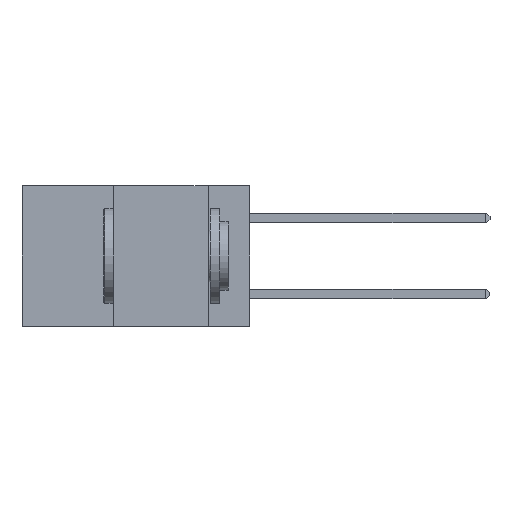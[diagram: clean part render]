
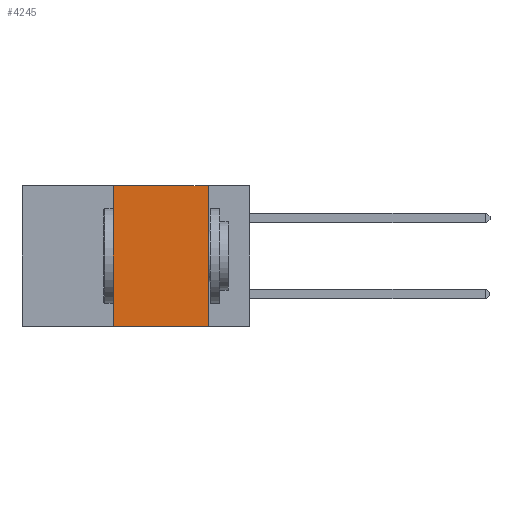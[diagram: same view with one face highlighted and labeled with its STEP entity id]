
A CAD part, left-side view. The second image highlights one B-rep face of the part: STEP entity #4245.
In plain terms, the highlighted planar face has unit normal (-1, 0, 0).
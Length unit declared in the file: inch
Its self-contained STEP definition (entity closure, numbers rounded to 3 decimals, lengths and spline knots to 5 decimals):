
#246 = CARTESIAN_POINT ( 'NONE',  ( 0., 0.11, -0.37 ) ) ;
#401 = DIRECTION ( 'NONE',  ( 0., 0., -1. ) ) ;
#532 = DIRECTION ( 'NONE',  ( 1., 0., 0. ) ) ;
#853 = CARTESIAN_POINT ( 'NONE',  ( 0., 0.6, -0.37 ) ) ;
#1138 = CARTESIAN_POINT ( 'NONE',  ( 0., 0.6, 0. ) ) ;
#1236 = PLANE ( 'NONE',  #7888 ) ;
#1429 = VECTOR ( 'NONE', #2829, 39.37008 ) ;
#1444 = VECTOR ( 'NONE', #10273, 39.37008 ) ;
#1738 = EDGE_LOOP ( 'NONE', ( #7374, #2840, #4292, #3475 ) ) ;
#2829 = DIRECTION ( 'NONE',  ( 0., 0., -1. ) ) ;
#2840 = ORIENTED_EDGE ( 'NONE', *, *, #3619, .F. ) ;
#3176 = VECTOR ( 'NONE', #3326, 39.37008 ) ;
#3211 = CARTESIAN_POINT ( 'NONE',  ( 0., 0.36, 0. ) ) ;
#3326 = DIRECTION ( 'NONE',  ( 0., -1., 0. ) ) ;
#3475 = ORIENTED_EDGE ( 'NONE', *, *, #9658, .T. ) ;
#3619 = EDGE_CURVE ( 'NONE', #6064, #11494, #4301, .T. ) ;
#3938 = VERTEX_POINT ( 'NONE', #13846 ) ;
#4157 = CARTESIAN_POINT ( 'NONE',  ( 0., 0.6, 0. ) ) ;
#4245 = ADVANCED_FACE ( 'NONE', ( #11407 ), #1236, .F. ) ;
#4252 = VERTEX_POINT ( 'NONE', #246 ) ;
#4292 = ORIENTED_EDGE ( 'NONE', *, *, #14094, .F. ) ;
#4301 = LINE ( 'NONE', #4157, #3176 ) ;
#4622 = LINE ( 'NONE', #853, #1444 ) ;
#6064 = VERTEX_POINT ( 'NONE', #11133 ) ;
#7374 = ORIENTED_EDGE ( 'NONE', *, *, #10111, .F. ) ;
#7888 = AXIS2_PLACEMENT_3D ( 'NONE', #1138, #532, #401 ) ;
#8120 = LINE ( 'NONE', #11054, #1429 ) ;
#9104 = DIRECTION ( 'NONE',  ( 0., 0., 1. ) ) ;
#9658 = EDGE_CURVE ( 'NONE', #3938, #4252, #4622, .T. ) ;
#10111 = EDGE_CURVE ( 'NONE', #11494, #4252, #8120, .T. ) ;
#10273 = DIRECTION ( 'NONE',  ( 0., -1., 0. ) ) ;
#10345 = LINE ( 'NONE', #3211, #12935 ) ;
#10732 = CARTESIAN_POINT ( 'NONE',  ( 0., 0.11, 0. ) ) ;
#11054 = CARTESIAN_POINT ( 'NONE',  ( 0., 0.11, 0. ) ) ;
#11133 = CARTESIAN_POINT ( 'NONE',  ( 0., 0.36, 0. ) ) ;
#11407 = FACE_OUTER_BOUND ( 'NONE', #1738, .T. ) ;
#11494 = VERTEX_POINT ( 'NONE', #10732 ) ;
#12935 = VECTOR ( 'NONE', #9104, 39.37008 ) ;
#13846 = CARTESIAN_POINT ( 'NONE',  ( 0., 0.36, -0.37 ) ) ;
#14094 = EDGE_CURVE ( 'NONE', #3938, #6064, #10345, .T. ) ;
